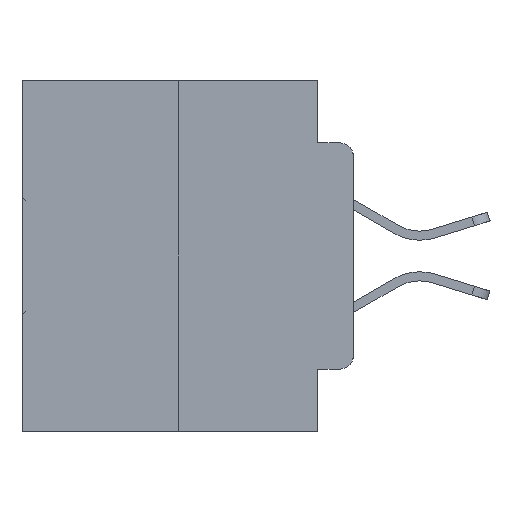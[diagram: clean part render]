
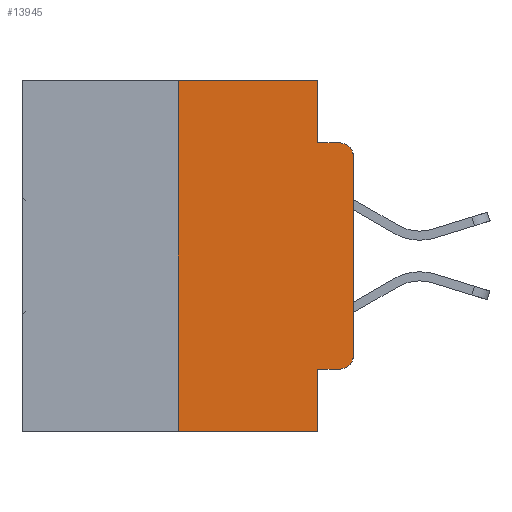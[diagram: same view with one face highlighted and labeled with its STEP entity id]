
A CAD part, left-side view. The second image highlights one B-rep face of the part: STEP entity #13945.
In plain terms, the highlighted planar face has unit normal (-1, 0, 0).
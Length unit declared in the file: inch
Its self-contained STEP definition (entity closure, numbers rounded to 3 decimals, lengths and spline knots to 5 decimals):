
#125 = LINE ( 'NONE', #316, #25860 ) ;
#160 = VERTEX_POINT ( 'NONE', #1104 ) ;
#316 = CARTESIAN_POINT ( 'NONE',  ( 0., 0.473, 0. ) ) ;
#569 = LINE ( 'NONE', #7050, #25908 ) ;
#1104 = CARTESIAN_POINT ( 'NONE',  ( 0., 0.02, -0.0885 ) ) ;
#1410 = CARTESIAN_POINT ( 'NONE',  ( 0., 0.02, -0.1085 ) ) ;
#2479 = LINE ( 'NONE', #11652, #20504 ) ;
#3124 = ORIENTED_EDGE ( 'NONE', *, *, #8258, .F. ) ;
#3901 = CARTESIAN_POINT ( 'NONE',  ( 0., 0.051, -0.0885 ) ) ;
#4214 = EDGE_CURVE ( 'NONE', #31085, #160, #31267, .T. ) ;
#4603 = CARTESIAN_POINT ( 'NONE',  ( 0., 0., -0.3915 ) ) ;
#4608 = DIRECTION ( 'NONE',  ( 0., -1., 0. ) ) ;
#4982 = VERTEX_POINT ( 'NONE', #24214 ) ;
#5169 = CIRCLE ( 'NONE', #26769, 0.02 ) ;
#5892 = CARTESIAN_POINT ( 'NONE',  ( 0., 0.051, 0. ) ) ;
#6472 = CARTESIAN_POINT ( 'NONE',  ( 0., 0., 0. ) ) ;
#6819 = CARTESIAN_POINT ( 'NONE',  ( 0., 0.051, -0.5 ) ) ;
#6830 = EDGE_CURVE ( 'NONE', #17898, #31144, #2479, .T. ) ;
#7050 = CARTESIAN_POINT ( 'NONE',  ( 0., 0.051, 0. ) ) ;
#7212 = VERTEX_POINT ( 'NONE', #6819 ) ;
#7339 = ORIENTED_EDGE ( 'NONE', *, *, #6830, .T. ) ;
#7365 = LINE ( 'NONE', #5892, #30357 ) ;
#8204 = PLANE ( 'NONE',  #16802 ) ;
#8258 = EDGE_CURVE ( 'NONE', #18698, #31085, #7365, .T. ) ;
#8489 = DIRECTION ( 'NONE',  ( 0., 0., -1. ) ) ;
#8810 = LINE ( 'NONE', #9107, #27977 ) ;
#9107 = CARTESIAN_POINT ( 'NONE',  ( 0., 0.473, -0.5 ) ) ;
#9664 = ORIENTED_EDGE ( 'NONE', *, *, #17185, .F. ) ;
#9889 = VECTOR ( 'NONE', #25215, 39.37008 ) ;
#10536 = EDGE_LOOP ( 'NONE', ( #11681, #20220, #30679, #3124, #31214, #9664, #22710, #21025, #7339, #25870 ) ) ;
#10735 = LINE ( 'NONE', #6472, #12644 ) ;
#11577 = DIRECTION ( 'NONE',  ( 0., -1., 0. ) ) ;
#11652 = CARTESIAN_POINT ( 'NONE',  ( 0., 0.051, -0.4115 ) ) ;
#11681 = ORIENTED_EDGE ( 'NONE', *, *, #28241, .T. ) ;
#11736 = DIRECTION ( 'NONE',  ( 0., 0., 1. ) ) ;
#12431 = VERTEX_POINT ( 'NONE', #30547 ) ;
#12644 = VECTOR ( 'NONE', #11736, 39.37008 ) ;
#12812 = EDGE_CURVE ( 'NONE', #31144, #13745, #22089, .T. ) ;
#12923 = CARTESIAN_POINT ( 'NONE',  ( 0., 0.25, 0. ) ) ;
#13357 = DIRECTION ( 'NONE',  ( -1., 0., 0. ) ) ;
#13497 = DIRECTION ( 'NONE',  ( 0., 0., -1. ) ) ;
#13745 = VERTEX_POINT ( 'NONE', #4603 ) ;
#13778 = DIRECTION ( 'NONE',  ( -1., 0., 0. ) ) ;
#13945 = ADVANCED_FACE ( 'NONE', ( #22393 ), #8204, .F. ) ;
#15445 = CARTESIAN_POINT ( 'NONE',  ( 0., 0.051, -0.4115 ) ) ;
#15838 = DIRECTION ( 'NONE',  ( 0., 0., -1. ) ) ;
#15940 = CARTESIAN_POINT ( 'NONE',  ( 0., 0.02, -0.3915 ) ) ;
#15958 = AXIS2_PLACEMENT_3D ( 'NONE', #15940, #13357, #15838 ) ;
#16309 = EDGE_CURVE ( 'NONE', #12431, #7212, #8810, .T. ) ;
#16802 = AXIS2_PLACEMENT_3D ( 'NONE', #18193, #23102, #13497 ) ;
#16891 = LINE ( 'NONE', #12923, #9889 ) ;
#17150 = DIRECTION ( 'NONE',  ( 0., 0., -1. ) ) ;
#17185 = EDGE_CURVE ( 'NONE', #12431, #26973, #16891, .T. ) ;
#17418 = DIRECTION ( 'NONE',  ( 0., -1., 0. ) ) ;
#17898 = VERTEX_POINT ( 'NONE', #15445 ) ;
#17914 = CARTESIAN_POINT ( 'NONE',  ( 0., 0.25, 0. ) ) ;
#18193 = CARTESIAN_POINT ( 'NONE',  ( 0., 0.473, 0. ) ) ;
#18698 = VERTEX_POINT ( 'NONE', #31127 ) ;
#19039 = DIRECTION ( 'NONE',  ( 0., -1., 0. ) ) ;
#20220 = ORIENTED_EDGE ( 'NONE', *, *, #21165, .T. ) ;
#20222 = EDGE_CURVE ( 'NONE', #17898, #7212, #569, .T. ) ;
#20504 = VECTOR ( 'NONE', #19039, 39.37008 ) ;
#21025 = ORIENTED_EDGE ( 'NONE', *, *, #20222, .F. ) ;
#21165 = EDGE_CURVE ( 'NONE', #4982, #160, #5169, .T. ) ;
#21845 = EDGE_CURVE ( 'NONE', #26973, #18698, #125, .T. ) ;
#22089 = CIRCLE ( 'NONE', #15958, 0.02 ) ;
#22393 = FACE_OUTER_BOUND ( 'NONE', #10536, .T. ) ;
#22710 = ORIENTED_EDGE ( 'NONE', *, *, #16309, .T. ) ;
#22927 = DIRECTION ( 'NONE',  ( 0., 0., -1. ) ) ;
#23102 = DIRECTION ( 'NONE',  ( 1., 0., 0. ) ) ;
#23902 = CARTESIAN_POINT ( 'NONE',  ( 0., 0.051, -0.0885 ) ) ;
#24214 = CARTESIAN_POINT ( 'NONE',  ( 0., 0., -0.1085 ) ) ;
#24755 = VECTOR ( 'NONE', #4608, 39.37008 ) ;
#25215 = DIRECTION ( 'NONE',  ( 0., 0., 1. ) ) ;
#25860 = VECTOR ( 'NONE', #17418, 39.37008 ) ;
#25870 = ORIENTED_EDGE ( 'NONE', *, *, #12812, .T. ) ;
#25908 = VECTOR ( 'NONE', #17150, 39.37008 ) ;
#26769 = AXIS2_PLACEMENT_3D ( 'NONE', #1410, #13778, #8489 ) ;
#26973 = VERTEX_POINT ( 'NONE', #17914 ) ;
#27977 = VECTOR ( 'NONE', #11577, 39.37008 ) ;
#28241 = EDGE_CURVE ( 'NONE', #13745, #4982, #10735, .T. ) ;
#30357 = VECTOR ( 'NONE', #22927, 39.37008 ) ;
#30547 = CARTESIAN_POINT ( 'NONE',  ( 0., 0.25, -0.5 ) ) ;
#30679 = ORIENTED_EDGE ( 'NONE', *, *, #4214, .F. ) ;
#31085 = VERTEX_POINT ( 'NONE', #3901 ) ;
#31127 = CARTESIAN_POINT ( 'NONE',  ( 0., 0.051, 0. ) ) ;
#31144 = VERTEX_POINT ( 'NONE', #31309 ) ;
#31214 = ORIENTED_EDGE ( 'NONE', *, *, #21845, .F. ) ;
#31267 = LINE ( 'NONE', #23902, #24755 ) ;
#31309 = CARTESIAN_POINT ( 'NONE',  ( 0., 0.02, -0.4115 ) ) ;
